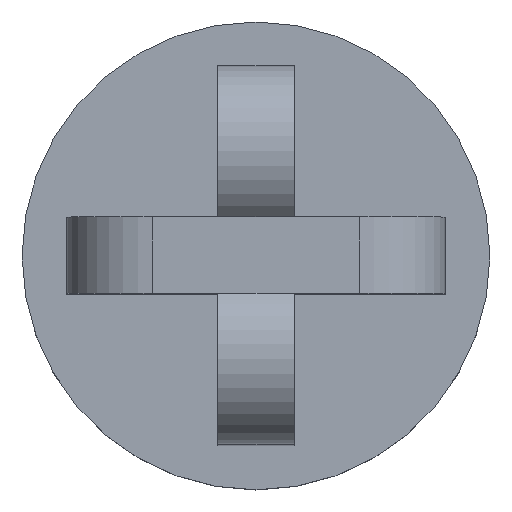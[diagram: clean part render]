
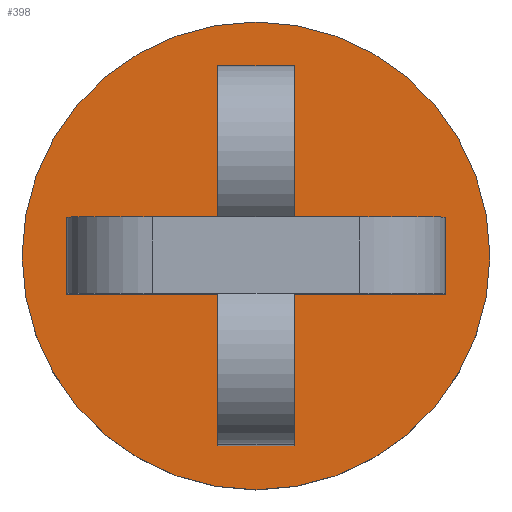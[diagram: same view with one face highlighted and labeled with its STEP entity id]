
A CAD part, top view. The second image highlights one B-rep face of the part: STEP entity #398.
In plain terms, the highlighted planar face has unit normal (0, 0, 1).
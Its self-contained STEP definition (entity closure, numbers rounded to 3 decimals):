
#15=FACE_BOUND('',#79,.T.);
#32=PLANE('',#450);
#55=FACE_OUTER_BOUND('',#78,.T.);
#78=EDGE_LOOP('',(#356));
#79=EDGE_LOOP('',(#357,#358,#359,#360,#361,#362,#363,#364,#365,#366,#367,
#368));
#85=LINE('',#582,#123);
#88=LINE('',#587,#126);
#89=LINE('',#590,#127);
#95=LINE('',#607,#133);
#104=LINE('',#627,#142);
#106=LINE('',#636,#144);
#109=LINE('',#641,#147);
#111=LINE('',#645,#149);
#112=LINE('',#647,#150);
#114=LINE('',#651,#152);
#116=LINE('',#655,#154);
#117=LINE('',#657,#155);
#123=VECTOR('',#465,10.);
#126=VECTOR('',#470,10.);
#127=VECTOR('',#473,10.);
#133=VECTOR('',#487,10.);
#142=VECTOR('',#506,10.);
#144=VECTOR('',#516,10.);
#147=VECTOR('',#521,10.);
#149=VECTOR('',#525,10.);
#150=VECTOR('',#528,10.);
#152=VECTOR('',#532,10.);
#154=VECTOR('',#536,10.);
#155=VECTOR('',#539,10.);
#172=CIRCLE('',#448,4.75);
#178=VERTEX_POINT('',#579);
#179=VERTEX_POINT('',#581);
#180=VERTEX_POINT('',#585);
#181=VERTEX_POINT('',#589);
#187=VERTEX_POINT('',#604);
#188=VERTEX_POINT('',#606);
#194=VERTEX_POINT('',#625);
#197=VERTEX_POINT('',#635);
#198=VERTEX_POINT('',#639);
#199=VERTEX_POINT('',#643);
#200=VERTEX_POINT('',#649);
#201=VERTEX_POINT('',#653);
#207=VERTEX_POINT('',#700);
#214=EDGE_CURVE('',#179,#178,#85,.T.);
#217=EDGE_CURVE('',#178,#180,#88,.T.);
#218=EDGE_CURVE('',#181,#179,#89,.T.);
#226=EDGE_CURVE('',#188,#187,#95,.T.);
#237=EDGE_CURVE('',#187,#194,#104,.T.);
#241=EDGE_CURVE('',#197,#181,#106,.T.);
#244=EDGE_CURVE('',#194,#198,#109,.T.);
#246=EDGE_CURVE('',#180,#199,#111,.T.);
#247=EDGE_CURVE('',#199,#188,#112,.T.);
#249=EDGE_CURVE('',#198,#200,#114,.T.);
#251=EDGE_CURVE('',#200,#201,#116,.T.);
#252=EDGE_CURVE('',#201,#197,#117,.T.);
#260=EDGE_CURVE('',#207,#207,#172,.T.);
#356=ORIENTED_EDGE('',*,*,#260,.T.);
#357=ORIENTED_EDGE('',*,*,#244,.T.);
#358=ORIENTED_EDGE('',*,*,#249,.T.);
#359=ORIENTED_EDGE('',*,*,#251,.T.);
#360=ORIENTED_EDGE('',*,*,#252,.T.);
#361=ORIENTED_EDGE('',*,*,#241,.T.);
#362=ORIENTED_EDGE('',*,*,#218,.T.);
#363=ORIENTED_EDGE('',*,*,#214,.T.);
#364=ORIENTED_EDGE('',*,*,#217,.T.);
#365=ORIENTED_EDGE('',*,*,#246,.T.);
#366=ORIENTED_EDGE('',*,*,#247,.T.);
#367=ORIENTED_EDGE('',*,*,#226,.T.);
#368=ORIENTED_EDGE('',*,*,#237,.T.);
#398=ADVANCED_FACE('',(#55,#15),#32,.T.);
#448=AXIS2_PLACEMENT_3D('',#701,#559,#560);
#450=AXIS2_PLACEMENT_3D('',#705,#564,#565);
#465=DIRECTION('',(1.,0.,0.));
#470=DIRECTION('',(0.,-1.,0.));
#473=DIRECTION('',(0.,1.,0.));
#487=DIRECTION('',(-1.,0.,0.));
#506=DIRECTION('',(0.,-1.,0.));
#516=DIRECTION('',(1.,0.,0.));
#521=DIRECTION('',(-1.,0.,0.));
#525=DIRECTION('',(1.,0.,0.));
#528=DIRECTION('',(0.,-1.,0.));
#532=DIRECTION('',(0.,1.,0.));
#536=DIRECTION('',(-1.,0.,0.));
#539=DIRECTION('',(0.,1.,0.));
#559=DIRECTION('center_axis',(0.,0.,1.));
#560=DIRECTION('ref_axis',(1.,0.,0.));
#564=DIRECTION('center_axis',(0.,0.,1.));
#565=DIRECTION('ref_axis',(1.,0.,0.));
#579=CARTESIAN_POINT('',(0.775,3.85,1.8));
#581=CARTESIAN_POINT('',(-0.775,3.85,1.8));
#582=CARTESIAN_POINT('',(0.388,3.85,1.8));
#585=CARTESIAN_POINT('',(0.775,0.775,1.8));
#587=CARTESIAN_POINT('',(0.775,0.388,1.8));
#589=CARTESIAN_POINT('',(-0.775,0.775,1.8));
#590=CARTESIAN_POINT('',(-0.775,1.925,1.8));
#604=CARTESIAN_POINT('',(0.775,-0.775,1.8));
#606=CARTESIAN_POINT('',(3.85,-0.775,1.8));
#607=CARTESIAN_POINT('',(0.388,-0.775,1.8));
#625=CARTESIAN_POINT('',(0.775,-3.85,1.8));
#627=CARTESIAN_POINT('',(0.775,-1.925,1.8));
#635=CARTESIAN_POINT('',(-3.85,0.775,1.8));
#636=CARTESIAN_POINT('',(-0.388,0.775,1.8));
#639=CARTESIAN_POINT('',(-0.775,-3.85,1.8));
#641=CARTESIAN_POINT('',(-0.388,-3.85,1.8));
#643=CARTESIAN_POINT('',(3.85,0.775,1.8));
#645=CARTESIAN_POINT('',(1.925,0.775,1.8));
#647=CARTESIAN_POINT('',(3.85,-0.388,1.8));
#649=CARTESIAN_POINT('',(-0.775,-0.775,1.8));
#651=CARTESIAN_POINT('',(-0.775,-0.388,1.8));
#653=CARTESIAN_POINT('',(-3.85,-0.775,1.8));
#655=CARTESIAN_POINT('',(-1.925,-0.775,1.8));
#657=CARTESIAN_POINT('',(-3.85,0.388,1.8));
#700=CARTESIAN_POINT('',(-4.75,0.,1.8));
#701=CARTESIAN_POINT('Origin',(0.,0.,1.8));
#705=CARTESIAN_POINT('Origin',(0.,0.,1.8));
